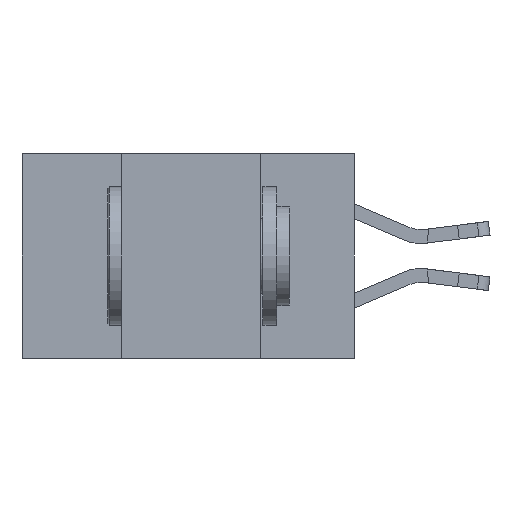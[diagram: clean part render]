
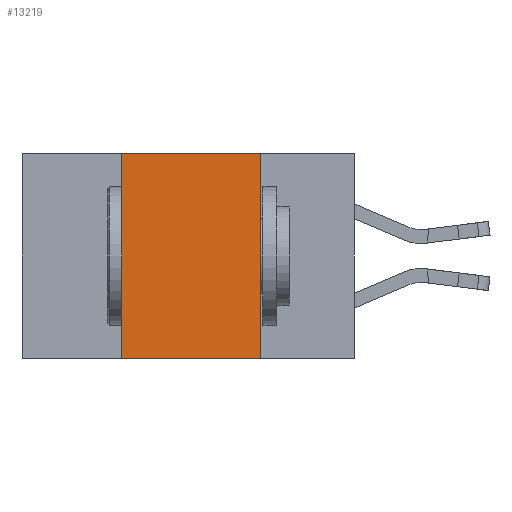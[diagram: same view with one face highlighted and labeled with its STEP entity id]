
A CAD part, left-side view. The second image highlights one B-rep face of the part: STEP entity #13219.
In plain terms, the highlighted planar face has unit normal (-1, 0, 0).
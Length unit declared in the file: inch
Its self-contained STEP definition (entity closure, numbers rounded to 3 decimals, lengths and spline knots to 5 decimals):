
#315 = EDGE_CURVE ( 'NONE', #3352, #13415, #14046, .T. ) ;
#1946 = VECTOR ( 'NONE', #10466, 39.37008 ) ;
#2562 = AXIS2_PLACEMENT_3D ( 'NONE', #21054, #6403, #6642 ) ;
#3171 = CARTESIAN_POINT ( 'NONE',  ( 0., 0.17, -0.37 ) ) ;
#3352 = VERTEX_POINT ( 'NONE', #3800 ) ;
#3800 = CARTESIAN_POINT ( 'NONE',  ( 0., 0.17, 0. ) ) ;
#5441 = CARTESIAN_POINT ( 'NONE',  ( 0., 0.17, -0.37 ) ) ;
#5650 = EDGE_LOOP ( 'NONE', ( #11607, #19112, #20191, #6456 ) ) ;
#6403 = DIRECTION ( 'NONE',  ( 1., 0., 0. ) ) ;
#6456 = ORIENTED_EDGE ( 'NONE', *, *, #10830, .T. ) ;
#6642 = DIRECTION ( 'NONE',  ( 0., 0., -1. ) ) ;
#8113 = EDGE_CURVE ( 'NONE', #18288, #3352, #21565, .T. ) ;
#8901 = DIRECTION ( 'NONE',  ( 0., -1., 0. ) ) ;
#9982 = FACE_OUTER_BOUND ( 'NONE', #5650, .T. ) ;
#10466 = DIRECTION ( 'NONE',  ( 0., 0., -1. ) ) ;
#10830 = EDGE_CURVE ( 'NONE', #12478, #13415, #21631, .T. ) ;
#11178 = DIRECTION ( 'NONE',  ( 0., -1., 0. ) ) ;
#11607 = ORIENTED_EDGE ( 'NONE', *, *, #315, .F. ) ;
#12377 = CARTESIAN_POINT ( 'NONE',  ( 0., 0.42, -0.37 ) ) ;
#12478 = VERTEX_POINT ( 'NONE', #17445 ) ;
#13219 = ADVANCED_FACE ( 'NONE', ( #9982 ), #22710, .F. ) ;
#13415 = VERTEX_POINT ( 'NONE', #5441 ) ;
#13627 = CARTESIAN_POINT ( 'NONE',  ( 0., 0.42, 0. ) ) ;
#14046 = LINE ( 'NONE', #3171, #1946 ) ;
#15821 = VECTOR ( 'NONE', #8901, 39.37008 ) ;
#15826 = LINE ( 'NONE', #12377, #18049 ) ;
#17113 = EDGE_CURVE ( 'NONE', #12478, #18288, #15826, .T. ) ;
#17445 = CARTESIAN_POINT ( 'NONE',  ( 0., 0.42, -0.37 ) ) ;
#17495 = DIRECTION ( 'NONE',  ( 0., 0., 1. ) ) ;
#18049 = VECTOR ( 'NONE', #17495, 39.37008 ) ;
#18288 = VERTEX_POINT ( 'NONE', #13627 ) ;
#18422 = CARTESIAN_POINT ( 'NONE',  ( 0., 0.6, 0. ) ) ;
#19112 = ORIENTED_EDGE ( 'NONE', *, *, #8113, .F. ) ;
#20191 = ORIENTED_EDGE ( 'NONE', *, *, #17113, .F. ) ;
#20743 = VECTOR ( 'NONE', #11178, 39.37008 ) ;
#21054 = CARTESIAN_POINT ( 'NONE',  ( 0., 0.6, 0. ) ) ;
#21513 = CARTESIAN_POINT ( 'NONE',  ( 0., 0.6, -0.37 ) ) ;
#21565 = LINE ( 'NONE', #18422, #20743 ) ;
#21631 = LINE ( 'NONE', #21513, #15821 ) ;
#22710 = PLANE ( 'NONE',  #2562 ) ;
